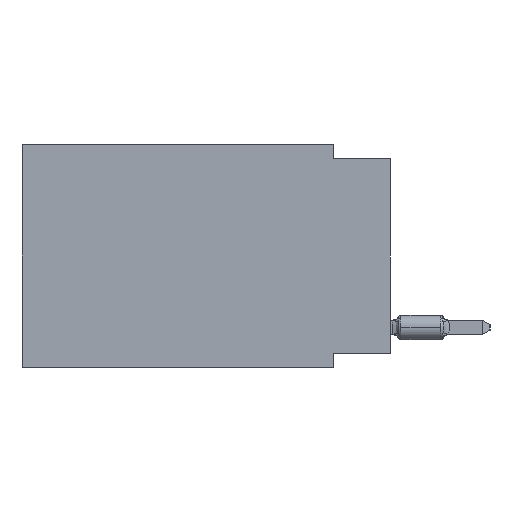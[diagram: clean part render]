
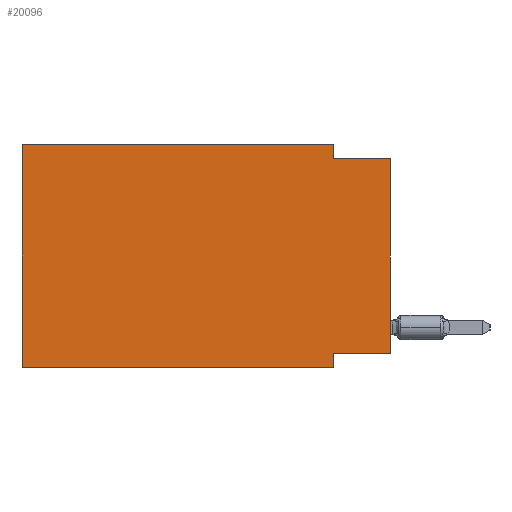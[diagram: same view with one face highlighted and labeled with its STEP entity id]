
A CAD part, left-side view. The second image highlights one B-rep face of the part: STEP entity #20096.
In plain terms, the highlighted planar face has unit normal (-1, 0, 0).
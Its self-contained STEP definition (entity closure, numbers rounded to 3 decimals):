
#238 = CARTESIAN_POINT ( 'NONE',  ( 0., 2.54, -9.271 ) ) ;
#922 = VERTEX_POINT ( 'NONE', #238 ) ;
#1581 = ORIENTED_EDGE ( 'NONE', *, *, #25993, .F. ) ;
#1799 = CARTESIAN_POINT ( 'NONE',  ( 0., 0., 0. ) ) ;
#2081 = CARTESIAN_POINT ( 'NONE',  ( 0., 2.54, -0.635 ) ) ;
#2963 = LINE ( 'NONE', #18764, #16441 ) ;
#2978 = DIRECTION ( 'NONE',  ( 0., 0., 1. ) ) ;
#3737 = CARTESIAN_POINT ( 'NONE',  ( 0., 16.383, 0. ) ) ;
#3867 = CARTESIAN_POINT ( 'NONE',  ( 0., 0., -9.271 ) ) ;
#4415 = CARTESIAN_POINT ( 'NONE',  ( 0., 16.383, -9.906 ) ) ;
#4514 = EDGE_CURVE ( 'NONE', #36580, #35150, #50802, .T. ) ;
#4580 = PLANE ( 'NONE',  #45726 ) ;
#4910 = VECTOR ( 'NONE', #12520, 1000. ) ;
#5087 = CARTESIAN_POINT ( 'NONE',  ( 0., 16.383, 0. ) ) ;
#5238 = VERTEX_POINT ( 'NONE', #2081 ) ;
#5517 = CARTESIAN_POINT ( 'NONE',  ( 0., 2.54, 0. ) ) ;
#5883 = LINE ( 'NONE', #49566, #29434 ) ;
#6771 = CARTESIAN_POINT ( 'NONE',  ( 0., 0., -0.635 ) ) ;
#7104 = ORIENTED_EDGE ( 'NONE', *, *, #50311, .F. ) ;
#7369 = DIRECTION ( 'NONE',  ( 0., -1., 0. ) ) ;
#7960 = VECTOR ( 'NONE', #13804, 1000. ) ;
#8236 = VECTOR ( 'NONE', #35823, 1000. ) ;
#8976 = EDGE_LOOP ( 'NONE', ( #36795, #7104, #1581, #19188, #26130, #22888, #33669, #45624 ) ) ;
#9171 = VERTEX_POINT ( 'NONE', #45145 ) ;
#9827 = LINE ( 'NONE', #1799, #22504 ) ;
#11342 = DIRECTION ( 'NONE',  ( 1., 0., 0. ) ) ;
#12520 = DIRECTION ( 'NONE',  ( 0., 0., -1. ) ) ;
#12850 = EDGE_CURVE ( 'NONE', #40162, #18692, #9827, .T. ) ;
#13804 = DIRECTION ( 'NONE',  ( 0., 0., -1. ) ) ;
#15483 = FACE_OUTER_BOUND ( 'NONE', #8976, .T. ) ;
#16441 = VECTOR ( 'NONE', #7369, 1000. ) ;
#17184 = LINE ( 'NONE', #5517, #4910 ) ;
#18692 = VERTEX_POINT ( 'NONE', #6771 ) ;
#18764 = CARTESIAN_POINT ( 'NONE',  ( 0., 16.383, -9.906 ) ) ;
#19014 = EDGE_CURVE ( 'NONE', #35150, #9171, #20368, .T. ) ;
#19188 = ORIENTED_EDGE ( 'NONE', *, *, #19014, .F. ) ;
#20096 = ADVANCED_FACE ( 'NONE', ( #15483 ), #4580, .F. ) ;
#20124 = CARTESIAN_POINT ( 'NONE',  ( 0., 16.383, 0. ) ) ;
#20368 = LINE ( 'NONE', #5087, #29291 ) ;
#21993 = DIRECTION ( 'NONE',  ( 0., 0., 1. ) ) ;
#22504 = VECTOR ( 'NONE', #21993, 1000. ) ;
#22888 = ORIENTED_EDGE ( 'NONE', *, *, #24742, .T. ) ;
#24742 = EDGE_CURVE ( 'NONE', #36580, #30375, #2963, .T. ) ;
#25993 = EDGE_CURVE ( 'NONE', #9171, #5238, #17184, .T. ) ;
#26130 = ORIENTED_EDGE ( 'NONE', *, *, #4514, .F. ) ;
#29291 = VECTOR ( 'NONE', #48766, 1000. ) ;
#29321 = LINE ( 'NONE', #45079, #7960 ) ;
#29346 = VECTOR ( 'NONE', #2978, 1000. ) ;
#29434 = VECTOR ( 'NONE', #33045, 1000. ) ;
#30375 = VERTEX_POINT ( 'NONE', #38916 ) ;
#32453 = LINE ( 'NONE', #48721, #8236 ) ;
#33045 = DIRECTION ( 'NONE',  ( 0., 1., 0. ) ) ;
#33669 = ORIENTED_EDGE ( 'NONE', *, *, #46873, .F. ) ;
#35150 = VERTEX_POINT ( 'NONE', #40106 ) ;
#35823 = DIRECTION ( 'NONE',  ( 0., -1., 0. ) ) ;
#36580 = VERTEX_POINT ( 'NONE', #4415 ) ;
#36795 = ORIENTED_EDGE ( 'NONE', *, *, #12850, .T. ) ;
#38916 = CARTESIAN_POINT ( 'NONE',  ( 0., 2.54, -9.906 ) ) ;
#40106 = CARTESIAN_POINT ( 'NONE',  ( 0., 16.383, 0. ) ) ;
#40162 = VERTEX_POINT ( 'NONE', #3867 ) ;
#43125 = DIRECTION ( 'NONE',  ( 0., 0., -1. ) ) ;
#44838 = EDGE_CURVE ( 'NONE', #40162, #922, #5883, .T. ) ;
#45079 = CARTESIAN_POINT ( 'NONE',  ( 0., 2.54, -9.906 ) ) ;
#45145 = CARTESIAN_POINT ( 'NONE',  ( 0., 2.54, 0. ) ) ;
#45624 = ORIENTED_EDGE ( 'NONE', *, *, #44838, .F. ) ;
#45726 = AXIS2_PLACEMENT_3D ( 'NONE', #20124, #11342, #43125 ) ;
#46873 = EDGE_CURVE ( 'NONE', #922, #30375, #29321, .T. ) ;
#48721 = CARTESIAN_POINT ( 'NONE',  ( 0., 0., -0.635 ) ) ;
#48766 = DIRECTION ( 'NONE',  ( 0., -1., 0. ) ) ;
#49566 = CARTESIAN_POINT ( 'NONE',  ( 0., 0., -9.271 ) ) ;
#50311 = EDGE_CURVE ( 'NONE', #5238, #18692, #32453, .T. ) ;
#50802 = LINE ( 'NONE', #3737, #29346 ) ;
